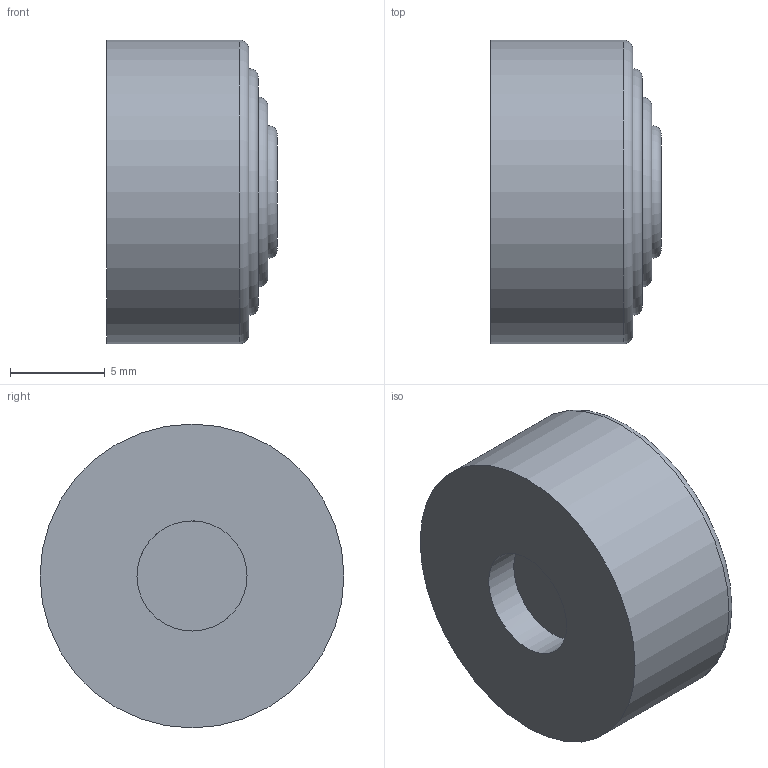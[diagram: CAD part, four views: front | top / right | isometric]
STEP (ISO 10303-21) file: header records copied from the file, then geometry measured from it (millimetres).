
FILE_DESCRIPTION (( 'STEP AP214' ), '1' );
FILE_NAME ('Mag_Release_Left_ButtonV0.1A.step', '2016-02-05T23:14:29', ( 'WarFairy' ), ( '' ), 'SwSTEP 2.0', 'SolidWorks 2015', '' );
FILE_SCHEMA (( 'AUTOMOTIVE_DESIGN' ));
Length unit declared in the file: millimetre
Products named in the file (1): Mag_Release_Left_ButtonV0.1A
Bounding box: 9 x 16 x 16 mm (x, y, z)
Volume: 1575.9 mm3; surface area: 828.8 mm2
Topology: 1 solids, 1 shells, 12 faces, 21 edges, 15 vertices
Faces by surface type: plane 6, torus 4, cylinder 2
Full cylindrical faces by diameter (mm): 5.8 x1, 16 x1
Entity records: 268 total; most frequent: DIRECTION 48, CARTESIAN_POINT 35, AXIS2_PLACEMENT_3D 24, ORIENTED_EDGE 22, EDGE_LOOP 22, FACE_OUTER_BOUND 18, ADVANCED_FACE 12, VERTEX_POINT 11
